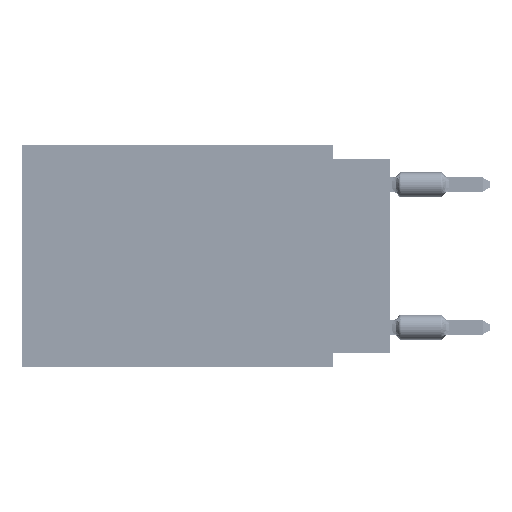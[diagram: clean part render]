
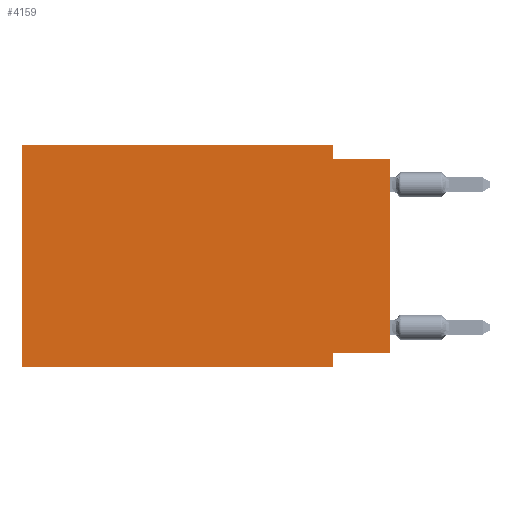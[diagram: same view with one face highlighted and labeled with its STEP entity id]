
A CAD part, left-side view. The second image highlights one B-rep face of the part: STEP entity #4159.
In plain terms, the highlighted planar face has unit normal (-1, 0, 0).
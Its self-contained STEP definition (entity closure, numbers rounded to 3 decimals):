
#1000 = VERTEX_POINT ( 'NONE', #5420 ) ;
#4159 = ADVANCED_FACE ( 'NONE', ( #81138 ), #48593, .F. ) ;
#4681 = VERTEX_POINT ( 'NONE', #17175 ) ;
#5420 = CARTESIAN_POINT ( 'NONE',  ( 0., 2.54, -9.906 ) ) ;
#6396 = EDGE_CURVE ( 'NONE', #31296, #1000, #69171, .T. ) ;
#6684 = EDGE_CURVE ( 'NONE', #72670, #63582, #35225, .T. ) ;
#9718 = CARTESIAN_POINT ( 'NONE',  ( 0., 0., -0.635 ) ) ;
#10066 = DIRECTION ( 'NONE',  ( 0., 0., -1. ) ) ;
#10651 = CARTESIAN_POINT ( 'NONE',  ( 0., 16.383, -9.906 ) ) ;
#11524 = LINE ( 'NONE', #10651, #27765 ) ;
#13028 = VECTOR ( 'NONE', #57098, 1000. ) ;
#13230 = VERTEX_POINT ( 'NONE', #81119 ) ;
#14971 = CARTESIAN_POINT ( 'NONE',  ( 0., 0., -9.271 ) ) ;
#16261 = EDGE_CURVE ( 'NONE', #72269, #13230, #16393, .T. ) ;
#16393 = LINE ( 'NONE', #30306, #82138 ) ;
#16925 = CARTESIAN_POINT ( 'NONE',  ( 0., 0., 0. ) ) ;
#17175 = CARTESIAN_POINT ( 'NONE',  ( 0., 2.54, -0.635 ) ) ;
#17607 = AXIS2_PLACEMENT_3D ( 'NONE', #54267, #53412, #79855 ) ;
#19129 = CARTESIAN_POINT ( 'NONE',  ( 0., 2.54, -9.271 ) ) ;
#19265 = VECTOR ( 'NONE', #10066, 1000. ) ;
#22449 = DIRECTION ( 'NONE',  ( 0., 0., -1. ) ) ;
#22450 = ORIENTED_EDGE ( 'NONE', *, *, #6396, .F. ) ;
#22549 = LINE ( 'NONE', #29083, #25349 ) ;
#23201 = DIRECTION ( 'NONE',  ( 0., 1., 0. ) ) ;
#23424 = ORIENTED_EDGE ( 'NONE', *, *, #6684, .T. ) ;
#23717 = DIRECTION ( 'NONE',  ( 0., -1., 0. ) ) ;
#24680 = CARTESIAN_POINT ( 'NONE',  ( 0., 0., -0.635 ) ) ;
#25349 = VECTOR ( 'NONE', #61644, 1000. ) ;
#27765 = VECTOR ( 'NONE', #23717, 1000. ) ;
#29083 = CARTESIAN_POINT ( 'NONE',  ( 0., 16.383, 0. ) ) ;
#29352 = EDGE_CURVE ( 'NONE', #13230, #59518, #22549, .T. ) ;
#30150 = EDGE_CURVE ( 'NONE', #59518, #4681, #75406, .T. ) ;
#30306 = CARTESIAN_POINT ( 'NONE',  ( 0., 16.383, 0. ) ) ;
#30623 = VECTOR ( 'NONE', #43419, 1000. ) ;
#30774 = EDGE_CURVE ( 'NONE', #4681, #63582, #69241, .T. ) ;
#31062 = VECTOR ( 'NONE', #22449, 1000. ) ;
#31296 = VERTEX_POINT ( 'NONE', #19129 ) ;
#35225 = LINE ( 'NONE', #16925, #30623 ) ;
#35406 = VECTOR ( 'NONE', #23201, 1000. ) ;
#35495 = ORIENTED_EDGE ( 'NONE', *, *, #72959, .F. ) ;
#36963 = ORIENTED_EDGE ( 'NONE', *, *, #16261, .F. ) ;
#43419 = DIRECTION ( 'NONE',  ( 0., 0., 1. ) ) ;
#43578 = ORIENTED_EDGE ( 'NONE', *, *, #30150, .F. ) ;
#47063 = CARTESIAN_POINT ( 'NONE',  ( 0., 2.54, 0. ) ) ;
#47752 = CARTESIAN_POINT ( 'NONE',  ( 0., 0., -9.271 ) ) ;
#48593 = PLANE ( 'NONE',  #17607 ) ;
#49622 = CARTESIAN_POINT ( 'NONE',  ( 0., 2.54, -9.906 ) ) ;
#51736 = EDGE_LOOP ( 'NONE', ( #23424, #61652, #43578, #69093, #36963, #85108, #22450, #35495 ) ) ;
#53412 = DIRECTION ( 'NONE',  ( 1., 0., 0. ) ) ;
#54267 = CARTESIAN_POINT ( 'NONE',  ( 0., 16.383, 0. ) ) ;
#55962 = DIRECTION ( 'NONE',  ( 0., 0., 1. ) ) ;
#57098 = DIRECTION ( 'NONE',  ( 0., -1., 0. ) ) ;
#59518 = VERTEX_POINT ( 'NONE', #47063 ) ;
#61130 = CARTESIAN_POINT ( 'NONE',  ( 0., 2.54, 0. ) ) ;
#61644 = DIRECTION ( 'NONE',  ( 0., -1., 0. ) ) ;
#61652 = ORIENTED_EDGE ( 'NONE', *, *, #30774, .F. ) ;
#63582 = VERTEX_POINT ( 'NONE', #24680 ) ;
#67853 = CARTESIAN_POINT ( 'NONE',  ( 0., 16.383, -9.906 ) ) ;
#68827 = LINE ( 'NONE', #14971, #35406 ) ;
#69093 = ORIENTED_EDGE ( 'NONE', *, *, #29352, .F. ) ;
#69171 = LINE ( 'NONE', #49622, #19265 ) ;
#69241 = LINE ( 'NONE', #9718, #13028 ) ;
#72269 = VERTEX_POINT ( 'NONE', #67853 ) ;
#72670 = VERTEX_POINT ( 'NONE', #47752 ) ;
#72959 = EDGE_CURVE ( 'NONE', #72670, #31296, #68827, .T. ) ;
#75406 = LINE ( 'NONE', #61130, #31062 ) ;
#79855 = DIRECTION ( 'NONE',  ( 0., 0., -1. ) ) ;
#81119 = CARTESIAN_POINT ( 'NONE',  ( 0., 16.383, 0. ) ) ;
#81138 = FACE_OUTER_BOUND ( 'NONE', #51736, .T. ) ;
#81401 = EDGE_CURVE ( 'NONE', #72269, #1000, #11524, .T. ) ;
#82138 = VECTOR ( 'NONE', #55962, 1000. ) ;
#85108 = ORIENTED_EDGE ( 'NONE', *, *, #81401, .T. ) ;
